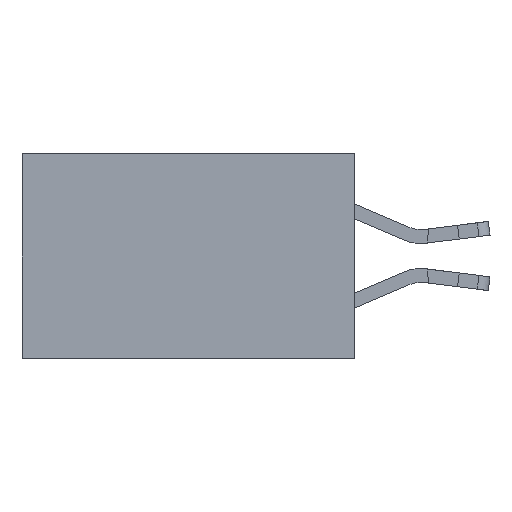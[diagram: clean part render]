
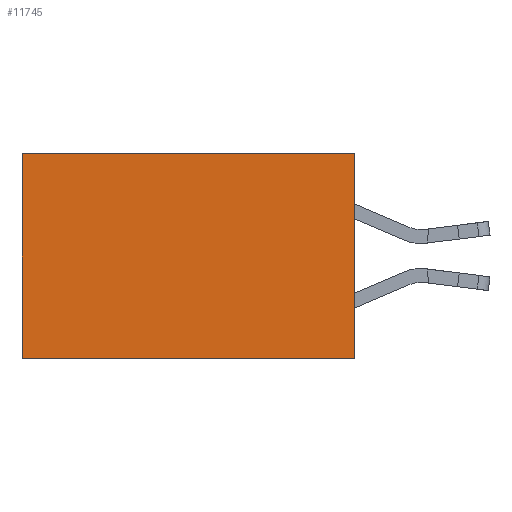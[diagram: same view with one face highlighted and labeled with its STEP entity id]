
A CAD part, left-side view. The second image highlights one B-rep face of the part: STEP entity #11745.
In plain terms, the highlighted planar face has unit normal (-1, 0, 0).
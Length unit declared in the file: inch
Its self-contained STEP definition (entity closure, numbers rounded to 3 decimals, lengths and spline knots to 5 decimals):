
#557 = VERTEX_POINT ( 'NONE', #8025 ) ;
#1960 = EDGE_CURVE ( 'NONE', #15435, #17798, #10028, .T. ) ;
#2307 = EDGE_CURVE ( 'NONE', #15435, #6229, #14334, .T. ) ;
#2507 = LINE ( 'NONE', #18242, #6999 ) ;
#2900 = VECTOR ( 'NONE', #16136, 39.37008 ) ;
#5396 = CARTESIAN_POINT ( 'NONE',  ( 0.2615, 0.6, -0.37 ) ) ;
#5688 = EDGE_CURVE ( 'NONE', #6229, #557, #8630, .T. ) ;
#6229 = VERTEX_POINT ( 'NONE', #7874 ) ;
#6371 = ORIENTED_EDGE ( 'NONE', *, *, #5688, .T. ) ;
#6901 = CARTESIAN_POINT ( 'NONE',  ( 0.2615, 0., -0.37 ) ) ;
#6999 = VECTOR ( 'NONE', #19555, 39.37008 ) ;
#7090 = CARTESIAN_POINT ( 'NONE',  ( 0.2615, 0., -0.37 ) ) ;
#7874 = CARTESIAN_POINT ( 'NONE',  ( 0.2615, 0.6, 0. ) ) ;
#8025 = CARTESIAN_POINT ( 'NONE',  ( 0.2615, 0.6, -0.37 ) ) ;
#8081 = DIRECTION ( 'NONE',  ( 1., 0., 0. ) ) ;
#8630 = LINE ( 'NONE', #5396, #18287 ) ;
#9186 = PLANE ( 'NONE',  #11175 ) ;
#10028 = LINE ( 'NONE', #7090, #2900 ) ;
#10924 = ORIENTED_EDGE ( 'NONE', *, *, #1960, .F. ) ;
#11175 = AXIS2_PLACEMENT_3D ( 'NONE', #17105, #8081, #17008 ) ;
#11317 = EDGE_LOOP ( 'NONE', ( #6371, #12326, #10924, #16866 ) ) ;
#11745 = ADVANCED_FACE ( 'NONE', ( #14002 ), #9186, .F. ) ;
#12326 = ORIENTED_EDGE ( 'NONE', *, *, #15209, .F. ) ;
#12933 = CARTESIAN_POINT ( 'NONE',  ( 0.2615, 0., 0. ) ) ;
#14002 = FACE_OUTER_BOUND ( 'NONE', #11317, .T. ) ;
#14334 = LINE ( 'NONE', #12933, #19065 ) ;
#14473 = DIRECTION ( 'NONE',  ( 0., 0., -1. ) ) ;
#15209 = EDGE_CURVE ( 'NONE', #17798, #557, #2507, .T. ) ;
#15435 = VERTEX_POINT ( 'NONE', #16806 ) ;
#15618 = DIRECTION ( 'NONE',  ( 0., 1., 0. ) ) ;
#16136 = DIRECTION ( 'NONE',  ( 0., 0., -1. ) ) ;
#16806 = CARTESIAN_POINT ( 'NONE',  ( 0.2615, 0., 0. ) ) ;
#16866 = ORIENTED_EDGE ( 'NONE', *, *, #2307, .T. ) ;
#17008 = DIRECTION ( 'NONE',  ( 0., 0., -1. ) ) ;
#17105 = CARTESIAN_POINT ( 'NONE',  ( 0.2615, 0., -0.37 ) ) ;
#17798 = VERTEX_POINT ( 'NONE', #6901 ) ;
#18242 = CARTESIAN_POINT ( 'NONE',  ( 0.2615, 0., -0.37 ) ) ;
#18287 = VECTOR ( 'NONE', #14473, 39.37008 ) ;
#19065 = VECTOR ( 'NONE', #15618, 39.37008 ) ;
#19555 = DIRECTION ( 'NONE',  ( 0., 1., 0. ) ) ;
